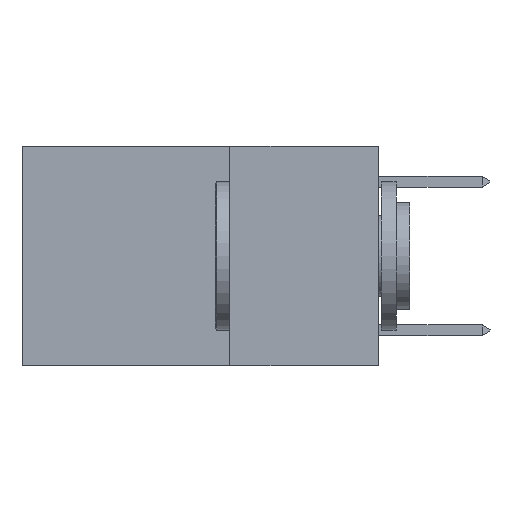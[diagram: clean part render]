
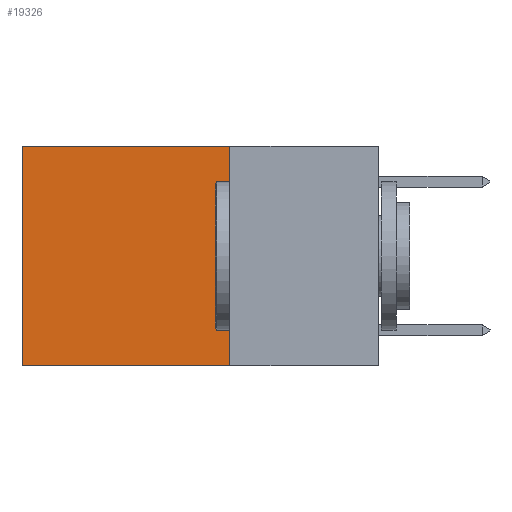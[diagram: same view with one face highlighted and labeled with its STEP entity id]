
A CAD part, left-side view. The second image highlights one B-rep face of the part: STEP entity #19326.
In plain terms, the highlighted planar face has unit normal (-1, 0, 0).
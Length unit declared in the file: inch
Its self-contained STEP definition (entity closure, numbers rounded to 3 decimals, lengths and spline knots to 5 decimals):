
#816 = EDGE_LOOP ( 'NONE', ( #16340, #13217, #8418, #19660 ) ) ;
#950 = CARTESIAN_POINT ( 'NONE',  ( 0.2625, 0.6, 0. ) ) ;
#1760 = DIRECTION ( 'NONE',  ( 0., 0., -1. ) ) ;
#2172 = EDGE_CURVE ( 'NONE', #2371, #29055, #29338, .T. ) ;
#2371 = VERTEX_POINT ( 'NONE', #8790 ) ;
#3242 = CARTESIAN_POINT ( 'NONE',  ( 0.2625, 0.25, 0. ) ) ;
#3319 = CARTESIAN_POINT ( 'NONE',  ( 0.2625, 0.6, 0. ) ) ;
#5480 = VERTEX_POINT ( 'NONE', #950 ) ;
#5604 = DIRECTION ( 'NONE',  ( 0., 1., 0. ) ) ;
#5722 = VECTOR ( 'NONE', #20957, 39.37008 ) ;
#5873 = DIRECTION ( 'NONE',  ( 0., 1., 0. ) ) ;
#6896 = CARTESIAN_POINT ( 'NONE',  ( 0.2625, 0.25, 0. ) ) ;
#7706 = AXIS2_PLACEMENT_3D ( 'NONE', #14216, #31506, #16772 ) ;
#8418 = ORIENTED_EDGE ( 'NONE', *, *, #17283, .F. ) ;
#8790 = CARTESIAN_POINT ( 'NONE',  ( 0.2625, 0.25, -0.37 ) ) ;
#9187 = CARTESIAN_POINT ( 'NONE',  ( 0.2625, 0.6, -0.37 ) ) ;
#10538 = EDGE_CURVE ( 'NONE', #18140, #5480, #27852, .T. ) ;
#13217 = ORIENTED_EDGE ( 'NONE', *, *, #2172, .F. ) ;
#14216 = CARTESIAN_POINT ( 'NONE',  ( 0.2625, 0.25, 0. ) ) ;
#16340 = ORIENTED_EDGE ( 'NONE', *, *, #24932, .T. ) ;
#16772 = DIRECTION ( 'NONE',  ( 0., 0., -1. ) ) ;
#17283 = EDGE_CURVE ( 'NONE', #18140, #2371, #23930, .T. ) ;
#18140 = VERTEX_POINT ( 'NONE', #29812 ) ;
#18281 = LINE ( 'NONE', #3319, #5722 ) ;
#18791 = FACE_OUTER_BOUND ( 'NONE', #816, .T. ) ;
#19326 = ADVANCED_FACE ( 'NONE', ( #18791 ), #26570, .F. ) ;
#19660 = ORIENTED_EDGE ( 'NONE', *, *, #10538, .T. ) ;
#20957 = DIRECTION ( 'NONE',  ( 0., 0., -1. ) ) ;
#23930 = LINE ( 'NONE', #6896, #29677 ) ;
#24932 = EDGE_CURVE ( 'NONE', #5480, #29055, #18281, .T. ) ;
#25640 = CARTESIAN_POINT ( 'NONE',  ( 0.2625, 0.25, -0.37 ) ) ;
#26570 = PLANE ( 'NONE',  #7706 ) ;
#27117 = VECTOR ( 'NONE', #5873, 39.37008 ) ;
#27852 = LINE ( 'NONE', #3242, #27117 ) ;
#29055 = VERTEX_POINT ( 'NONE', #9187 ) ;
#29338 = LINE ( 'NONE', #25640, #29363 ) ;
#29363 = VECTOR ( 'NONE', #5604, 39.37008 ) ;
#29677 = VECTOR ( 'NONE', #1760, 39.37008 ) ;
#29812 = CARTESIAN_POINT ( 'NONE',  ( 0.2625, 0.25, 0. ) ) ;
#31506 = DIRECTION ( 'NONE',  ( 1., 0., 0. ) ) ;
